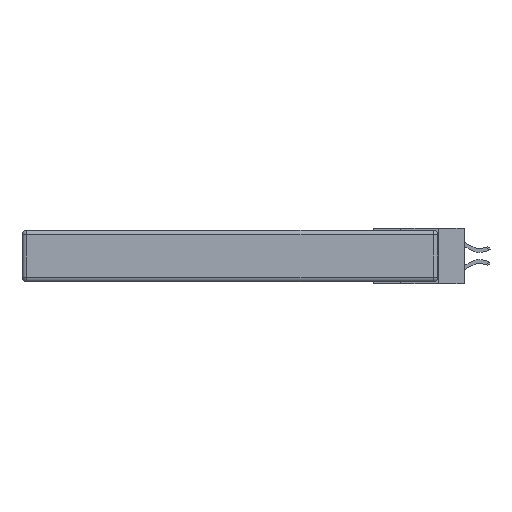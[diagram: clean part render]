
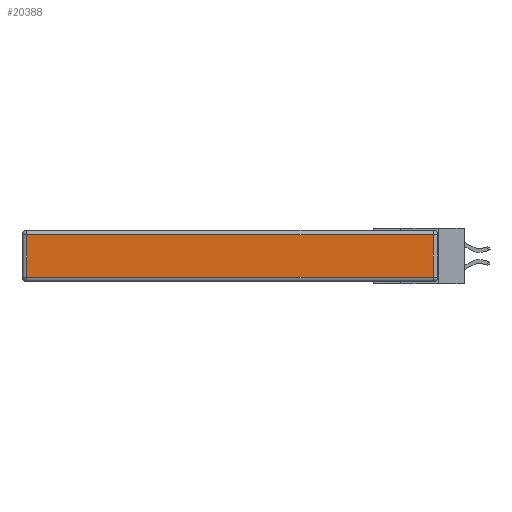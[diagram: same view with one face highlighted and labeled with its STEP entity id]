
A CAD part, left-side view. The second image highlights one B-rep face of the part: STEP entity #20388.
In plain terms, the highlighted planar face has unit normal (-1, 0, 0).
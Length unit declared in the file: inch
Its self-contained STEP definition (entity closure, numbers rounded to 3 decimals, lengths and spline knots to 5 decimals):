
#582 = CARTESIAN_POINT ( 'NONE',  ( 0., 2.75, -0.03 ) ) ;
#1118 = LINE ( 'NONE', #21631, #20417 ) ;
#1166 = DIRECTION ( 'NONE',  ( -1., 0., 0. ) ) ;
#2852 = AXIS2_PLACEMENT_3D ( 'NONE', #31457, #1166, #6251 ) ;
#5638 = CARTESIAN_POINT ( 'NONE',  ( 0., 0.03, -0.313 ) ) ;
#5823 = ORIENTED_EDGE ( 'NONE', *, *, #31977, .T. ) ;
#6251 = DIRECTION ( 'NONE',  ( 0., 0., 1. ) ) ;
#6839 = EDGE_LOOP ( 'NONE', ( #19527, #29665, #30538, #5823 ) ) ;
#8978 = LINE ( 'NONE', #25493, #32439 ) ;
#10000 = DIRECTION ( 'NONE',  ( 0., -1., 0. ) ) ;
#10195 = DIRECTION ( 'NONE',  ( 0., 0., -1. ) ) ;
#14639 = VERTEX_POINT ( 'NONE', #31962 ) ;
#17357 = LINE ( 'NONE', #24975, #25932 ) ;
#17433 = EDGE_CURVE ( 'NONE', #22103, #14639, #1118, .T. ) ;
#19527 = ORIENTED_EDGE ( 'NONE', *, *, #25606, .T. ) ;
#19891 = CARTESIAN_POINT ( 'NONE',  ( 0., 2.72, -0.313 ) ) ;
#20388 = ADVANCED_FACE ( 'NONE', ( #29182 ), #28546, .T. ) ;
#20417 = VECTOR ( 'NONE', #21196, 39.37008 ) ;
#21196 = DIRECTION ( 'NONE',  ( 0., 0., 1. ) ) ;
#21631 = CARTESIAN_POINT ( 'NONE',  ( 0., 0.03, -0.343 ) ) ;
#21861 = EDGE_CURVE ( 'NONE', #14639, #26199, #31876, .T. ) ;
#22103 = VERTEX_POINT ( 'NONE', #5638 ) ;
#24975 = CARTESIAN_POINT ( 'NONE',  ( 0., 0., -0.313 ) ) ;
#25100 = VERTEX_POINT ( 'NONE', #19891 ) ;
#25493 = CARTESIAN_POINT ( 'NONE',  ( 0., 2.72, -0.343 ) ) ;
#25606 = EDGE_CURVE ( 'NONE', #25100, #22103, #17357, .T. ) ;
#25932 = VECTOR ( 'NONE', #10000, 39.37008 ) ;
#26199 = VERTEX_POINT ( 'NONE', #26632 ) ;
#26253 = DIRECTION ( 'NONE',  ( 0., 1., 0. ) ) ;
#26632 = CARTESIAN_POINT ( 'NONE',  ( 0., 2.72, -0.03 ) ) ;
#28546 = PLANE ( 'NONE',  #2852 ) ;
#29182 = FACE_OUTER_BOUND ( 'NONE', #6839, .T. ) ;
#29665 = ORIENTED_EDGE ( 'NONE', *, *, #17433, .T. ) ;
#30538 = ORIENTED_EDGE ( 'NONE', *, *, #21861, .T. ) ;
#30701 = VECTOR ( 'NONE', #26253, 39.37008 ) ;
#31457 = CARTESIAN_POINT ( 'NONE',  ( 0., 0., -0.343 ) ) ;
#31876 = LINE ( 'NONE', #582, #30701 ) ;
#31962 = CARTESIAN_POINT ( 'NONE',  ( 0., 0.03, -0.03 ) ) ;
#31977 = EDGE_CURVE ( 'NONE', #26199, #25100, #8978, .T. ) ;
#32439 = VECTOR ( 'NONE', #10195, 39.37008 ) ;
